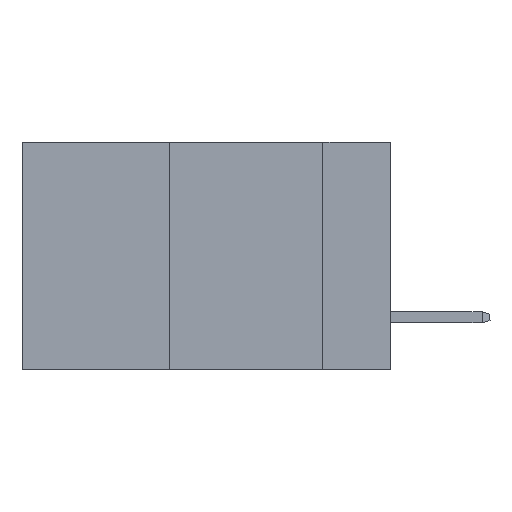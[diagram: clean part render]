
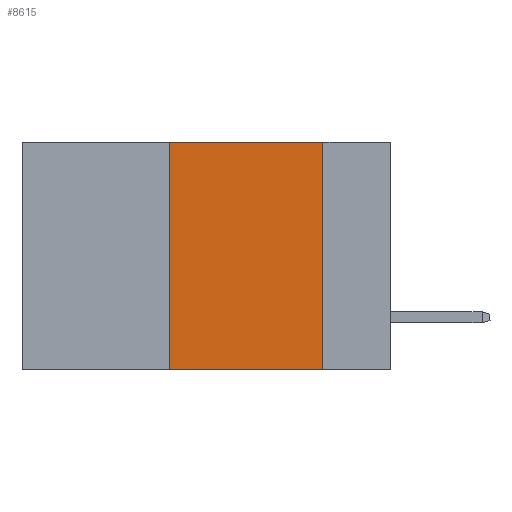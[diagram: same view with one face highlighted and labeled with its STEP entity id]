
A CAD part, left-side view. The second image highlights one B-rep face of the part: STEP entity #8615.
In plain terms, the highlighted planar face has unit normal (-1, 0, 0).
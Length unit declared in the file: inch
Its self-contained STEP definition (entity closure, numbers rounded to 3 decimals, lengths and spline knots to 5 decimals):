
#2057 = DIRECTION ( 'NONE',  ( 0., -1., 0. ) ) ;
#3264 = LINE ( 'NONE', #4169, #17754 ) ;
#4169 = CARTESIAN_POINT ( 'NONE',  ( 0., 0.6, -0.37 ) ) ;
#4890 = LINE ( 'NONE', #19917, #18521 ) ;
#5307 = LINE ( 'NONE', #15665, #6173 ) ;
#5796 = FACE_OUTER_BOUND ( 'NONE', #22262, .T. ) ;
#6173 = VECTOR ( 'NONE', #2057, 39.37008 ) ;
#6339 = DIRECTION ( 'NONE',  ( 0., 0., 1. ) ) ;
#7325 = ORIENTED_EDGE ( 'NONE', *, *, #14326, .T. ) ;
#7457 = EDGE_CURVE ( 'NONE', #10743, #15240, #4890, .T. ) ;
#8615 = ADVANCED_FACE ( 'NONE', ( #5796 ), #28045, .F. ) ;
#9421 = ORIENTED_EDGE ( 'NONE', *, *, #33621, .F. ) ;
#10065 = DIRECTION ( 'NONE',  ( 0., 0., -1. ) ) ;
#10743 = VERTEX_POINT ( 'NONE', #24573 ) ;
#11850 = DIRECTION ( 'NONE',  ( 1., 0., 0. ) ) ;
#13027 = VERTEX_POINT ( 'NONE', #31502 ) ;
#14326 = EDGE_CURVE ( 'NONE', #10743, #30875, #3264, .T. ) ;
#15240 = VERTEX_POINT ( 'NONE', #21932 ) ;
#15665 = CARTESIAN_POINT ( 'NONE',  ( 0., 0.6, 0. ) ) ;
#17754 = VECTOR ( 'NONE', #23170, 39.37008 ) ;
#18132 = VECTOR ( 'NONE', #10065, 39.37008 ) ;
#18521 = VECTOR ( 'NONE', #6339, 39.37008 ) ;
#19917 = CARTESIAN_POINT ( 'NONE',  ( 0., 0.36, 0. ) ) ;
#21932 = CARTESIAN_POINT ( 'NONE',  ( 0., 0.36, 0. ) ) ;
#22262 = EDGE_LOOP ( 'NONE', ( #33759, #9421, #26388, #7325 ) ) ;
#23170 = DIRECTION ( 'NONE',  ( 0., -1., 0. ) ) ;
#24573 = CARTESIAN_POINT ( 'NONE',  ( 0., 0.36, -0.37 ) ) ;
#26288 = CARTESIAN_POINT ( 'NONE',  ( 0., 0.11, 0. ) ) ;
#26388 = ORIENTED_EDGE ( 'NONE', *, *, #7457, .F. ) ;
#28045 = PLANE ( 'NONE',  #32525 ) ;
#30599 = CARTESIAN_POINT ( 'NONE',  ( 0., 0.6, 0. ) ) ;
#30705 = DIRECTION ( 'NONE',  ( 0., 0., -1. ) ) ;
#30875 = VERTEX_POINT ( 'NONE', #31041 ) ;
#31003 = EDGE_CURVE ( 'NONE', #13027, #30875, #33140, .T. ) ;
#31041 = CARTESIAN_POINT ( 'NONE',  ( 0., 0.11, -0.37 ) ) ;
#31502 = CARTESIAN_POINT ( 'NONE',  ( 0., 0.11, 0. ) ) ;
#32525 = AXIS2_PLACEMENT_3D ( 'NONE', #30599, #11850, #30705 ) ;
#33140 = LINE ( 'NONE', #26288, #18132 ) ;
#33621 = EDGE_CURVE ( 'NONE', #15240, #13027, #5307, .T. ) ;
#33759 = ORIENTED_EDGE ( 'NONE', *, *, #31003, .F. ) ;
